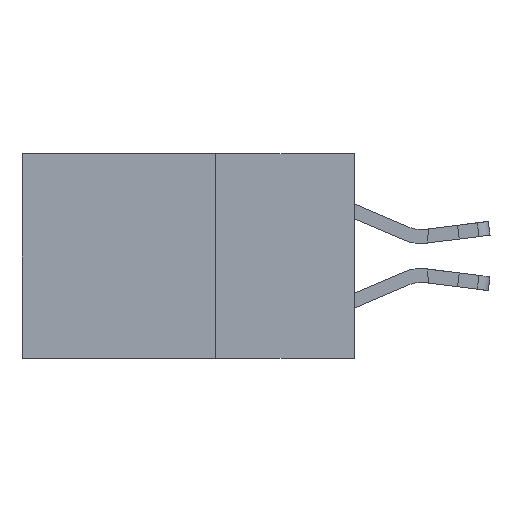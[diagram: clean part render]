
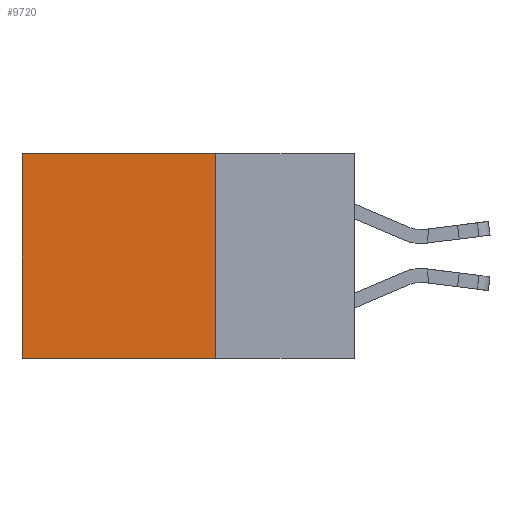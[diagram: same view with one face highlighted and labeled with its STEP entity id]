
A CAD part, left-side view. The second image highlights one B-rep face of the part: STEP entity #9720.
In plain terms, the highlighted planar face has unit normal (-1, 0, 0).
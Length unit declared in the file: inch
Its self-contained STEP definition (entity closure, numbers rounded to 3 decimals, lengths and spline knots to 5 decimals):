
#425 = LINE ( 'NONE', #5660, #13882 ) ;
#595 = DIRECTION ( 'NONE',  ( 0., 1., 0. ) ) ;
#859 = VERTEX_POINT ( 'NONE', #4581 ) ;
#1068 = PLANE ( 'NONE',  #6710 ) ;
#2117 = CARTESIAN_POINT ( 'NONE',  ( 0.2615, 0.25, -0.37 ) ) ;
#2759 = CARTESIAN_POINT ( 'NONE',  ( 0.2615, 0.25, -0.37 ) ) ;
#3265 = VECTOR ( 'NONE', #16788, 39.37008 ) ;
#4389 = VECTOR ( 'NONE', #7116, 39.37008 ) ;
#4581 = CARTESIAN_POINT ( 'NONE',  ( 0.2615, 0.6, 0. ) ) ;
#4686 = EDGE_LOOP ( 'NONE', ( #15765, #10106, #5896, #17070 ) ) ;
#4727 = LINE ( 'NONE', #8860, #3265 ) ;
#4809 = VERTEX_POINT ( 'NONE', #8053 ) ;
#5527 = VECTOR ( 'NONE', #15374, 39.37008 ) ;
#5660 = CARTESIAN_POINT ( 'NONE',  ( 0.2615, 0.25, -0.37 ) ) ;
#5896 = ORIENTED_EDGE ( 'NONE', *, *, #13095, .F. ) ;
#6710 = AXIS2_PLACEMENT_3D ( 'NONE', #2117, #9100, #7544 ) ;
#7038 = LINE ( 'NONE', #2759, #4389 ) ;
#7116 = DIRECTION ( 'NONE',  ( 0., 0., -1. ) ) ;
#7544 = DIRECTION ( 'NONE',  ( 0., 0., -1. ) ) ;
#8053 = CARTESIAN_POINT ( 'NONE',  ( 0.2615, 0.25, -0.37 ) ) ;
#8059 = EDGE_CURVE ( 'NONE', #859, #16595, #12638, .T. ) ;
#8851 = FACE_OUTER_BOUND ( 'NONE', #4686, .T. ) ;
#8860 = CARTESIAN_POINT ( 'NONE',  ( 0.2615, 0.25, 0. ) ) ;
#9100 = DIRECTION ( 'NONE',  ( 1., 0., 0. ) ) ;
#9720 = ADVANCED_FACE ( 'NONE', ( #8851 ), #1068, .F. ) ;
#10106 = ORIENTED_EDGE ( 'NONE', *, *, #12924, .F. ) ;
#11393 = CARTESIAN_POINT ( 'NONE',  ( 0.2615, 0.6, -0.37 ) ) ;
#12638 = LINE ( 'NONE', #13884, #5527 ) ;
#12924 = EDGE_CURVE ( 'NONE', #4809, #16595, #425, .T. ) ;
#13095 = EDGE_CURVE ( 'NONE', #15026, #4809, #7038, .T. ) ;
#13218 = EDGE_CURVE ( 'NONE', #15026, #859, #4727, .T. ) ;
#13882 = VECTOR ( 'NONE', #595, 39.37008 ) ;
#13884 = CARTESIAN_POINT ( 'NONE',  ( 0.2615, 0.6, -0.37 ) ) ;
#15026 = VERTEX_POINT ( 'NONE', #16179 ) ;
#15374 = DIRECTION ( 'NONE',  ( 0., 0., -1. ) ) ;
#15765 = ORIENTED_EDGE ( 'NONE', *, *, #8059, .T. ) ;
#16179 = CARTESIAN_POINT ( 'NONE',  ( 0.2615, 0.25, 0. ) ) ;
#16595 = VERTEX_POINT ( 'NONE', #11393 ) ;
#16788 = DIRECTION ( 'NONE',  ( 0., 1., 0. ) ) ;
#17070 = ORIENTED_EDGE ( 'NONE', *, *, #13218, .T. ) ;
